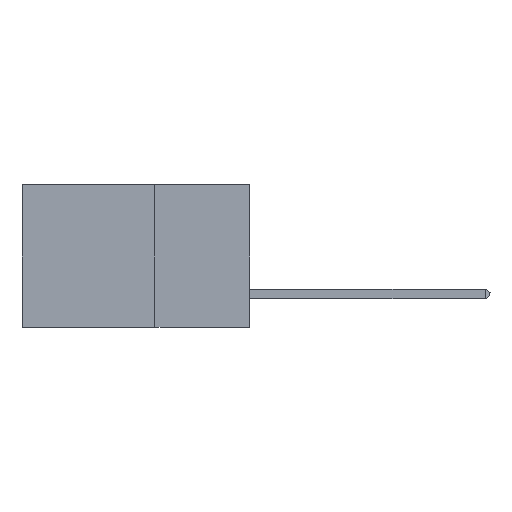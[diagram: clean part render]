
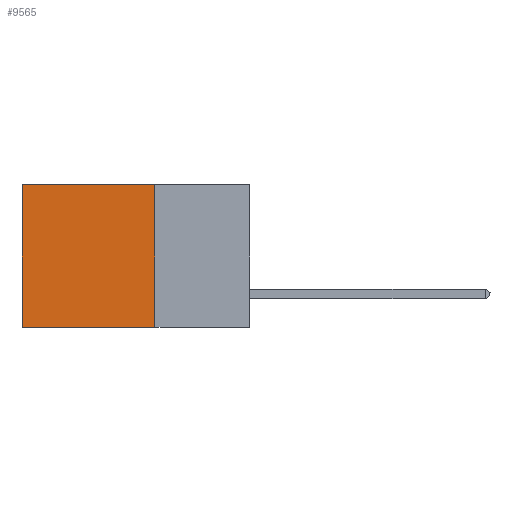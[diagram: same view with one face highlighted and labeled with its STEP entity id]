
A CAD part, left-side view. The second image highlights one B-rep face of the part: STEP entity #9565.
In plain terms, the highlighted planar face has unit normal (-1, 0, 0).
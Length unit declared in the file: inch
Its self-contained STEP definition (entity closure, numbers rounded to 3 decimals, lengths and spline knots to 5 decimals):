
#215 = VERTEX_POINT ( 'NONE', #6192 ) ;
#271 = LINE ( 'NONE', #13082, #12596 ) ;
#371 = DIRECTION ( 'NONE',  ( 0., 0., -1. ) ) ;
#2200 = CARTESIAN_POINT ( 'NONE',  ( 0.2875, 0.25, 0. ) ) ;
#2203 = ORIENTED_EDGE ( 'NONE', *, *, #7914, .F. ) ;
#3663 = DIRECTION ( 'NONE',  ( 0., 1., 0. ) ) ;
#4387 = PLANE ( 'NONE',  #11795 ) ;
#5120 = CARTESIAN_POINT ( 'NONE',  ( 0.2875, 0.6, -0.375 ) ) ;
#5423 = EDGE_CURVE ( 'NONE', #13084, #7393, #271, .T. ) ;
#6028 = DIRECTION ( 'NONE',  ( 0., 1., 0. ) ) ;
#6192 = CARTESIAN_POINT ( 'NONE',  ( 0.2875, 0.6, 0. ) ) ;
#7392 = VECTOR ( 'NONE', #13255, 39.37008 ) ;
#7393 = VERTEX_POINT ( 'NONE', #17864 ) ;
#7532 = DIRECTION ( 'NONE',  ( 0., 0., -1. ) ) ;
#7871 = EDGE_LOOP ( 'NONE', ( #11650, #17966, #2203, #13325 ) ) ;
#7914 = EDGE_CURVE ( 'NONE', #7939, #13084, #13513, .T. ) ;
#7939 = VERTEX_POINT ( 'NONE', #2200 ) ;
#8769 = EDGE_CURVE ( 'NONE', #7939, #215, #15980, .T. ) ;
#9565 = ADVANCED_FACE ( 'NONE', ( #10941 ), #4387, .F. ) ;
#10941 = FACE_OUTER_BOUND ( 'NONE', #7871, .T. ) ;
#11650 = ORIENTED_EDGE ( 'NONE', *, *, #18884, .T. ) ;
#11795 = AXIS2_PLACEMENT_3D ( 'NONE', #19049, #17497, #7532 ) ;
#12596 = VECTOR ( 'NONE', #3663, 39.37008 ) ;
#13082 = CARTESIAN_POINT ( 'NONE',  ( 0.2875, 0.25, -0.375 ) ) ;
#13084 = VERTEX_POINT ( 'NONE', #20762 ) ;
#13197 = LINE ( 'NONE', #5120, #7392 ) ;
#13255 = DIRECTION ( 'NONE',  ( 0., 0., -1. ) ) ;
#13306 = CARTESIAN_POINT ( 'NONE',  ( 0.2875, 0.25, -0.375 ) ) ;
#13325 = ORIENTED_EDGE ( 'NONE', *, *, #8769, .T. ) ;
#13513 = LINE ( 'NONE', #13306, #20567 ) ;
#14038 = CARTESIAN_POINT ( 'NONE',  ( 0.2875, 0.25, 0. ) ) ;
#14480 = VECTOR ( 'NONE', #6028, 39.37008 ) ;
#15980 = LINE ( 'NONE', #14038, #14480 ) ;
#17497 = DIRECTION ( 'NONE',  ( 1., 0., 0. ) ) ;
#17864 = CARTESIAN_POINT ( 'NONE',  ( 0.2875, 0.6, -0.375 ) ) ;
#17966 = ORIENTED_EDGE ( 'NONE', *, *, #5423, .F. ) ;
#18884 = EDGE_CURVE ( 'NONE', #215, #7393, #13197, .T. ) ;
#19049 = CARTESIAN_POINT ( 'NONE',  ( 0.2875, 0.25, -0.375 ) ) ;
#20567 = VECTOR ( 'NONE', #371, 39.37008 ) ;
#20762 = CARTESIAN_POINT ( 'NONE',  ( 0.2875, 0.25, -0.375 ) ) ;
